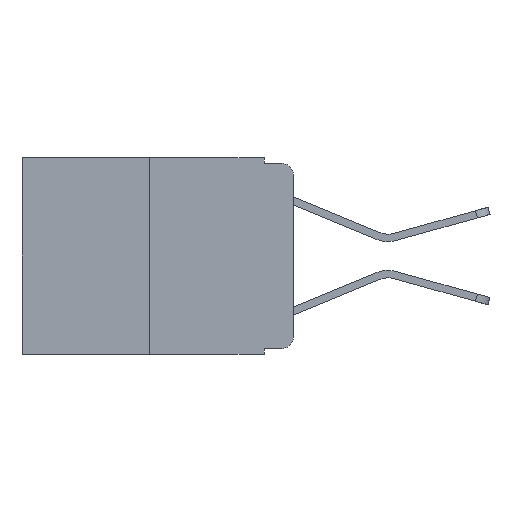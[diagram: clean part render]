
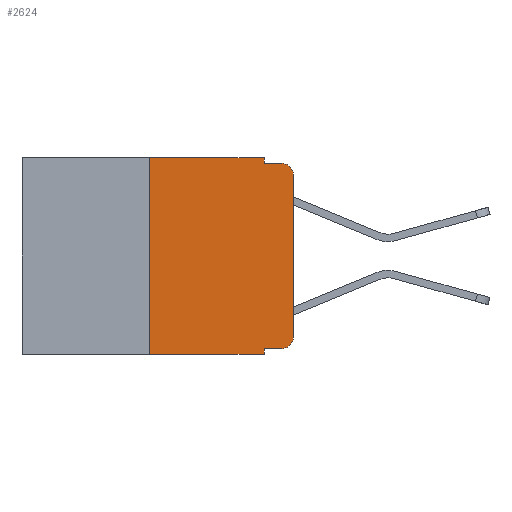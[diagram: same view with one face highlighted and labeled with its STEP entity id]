
A CAD part, left-side view. The second image highlights one B-rep face of the part: STEP entity #2624.
In plain terms, the highlighted planar face has unit normal (-1, 0, 0).
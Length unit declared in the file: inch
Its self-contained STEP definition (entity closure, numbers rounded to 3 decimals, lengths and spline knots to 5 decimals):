
#19 = ORIENTED_EDGE ( 'NONE', *, *, #8241, .F. ) ;
#22 = VECTOR ( 'NONE', #1344, 39.37008 ) ;
#104 = DIRECTION ( 'NONE',  ( 0., 0., -1. ) ) ;
#191 = ORIENTED_EDGE ( 'NONE', *, *, #8265, .F. ) ;
#260 = VERTEX_POINT ( 'NONE', #2706 ) ;
#266 = AXIS2_PLACEMENT_3D ( 'NONE', #10772, #7890, #8023 ) ;
#267 = VERTEX_POINT ( 'NONE', #2724 ) ;
#391 = LINE ( 'NONE', #6161, #5892 ) ;
#557 = ORIENTED_EDGE ( 'NONE', *, *, #8299, .T. ) ;
#726 = LINE ( 'NONE', #6759, #3659 ) ;
#813 = VERTEX_POINT ( 'NONE', #11244 ) ;
#1041 = FACE_OUTER_BOUND ( 'NONE', #6164, .T. ) ;
#1208 = CARTESIAN_POINT ( 'NONE',  ( 0., 0.25, 0. ) ) ;
#1344 = DIRECTION ( 'NONE',  ( 0., 0., 1. ) ) ;
#1414 = VECTOR ( 'NONE', #2322, 39.37008 ) ;
#1485 = EDGE_CURVE ( 'NONE', #267, #6537, #5308, .T. ) ;
#2110 = LINE ( 'NONE', #6670, #7257 ) ;
#2287 = VECTOR ( 'NONE', #10143, 39.37008 ) ;
#2322 = DIRECTION ( 'NONE',  ( 0., 0., 1. ) ) ;
#2362 = CARTESIAN_POINT ( 'NONE',  ( 0., 0.02, -0.313 ) ) ;
#2624 = ADVANCED_FACE ( 'NONE', ( #1041 ), #6940, .F. ) ;
#2632 = LINE ( 'NONE', #9280, #2287 ) ;
#2706 = CARTESIAN_POINT ( 'NONE',  ( 0., 0.02, -0.333 ) ) ;
#2724 = CARTESIAN_POINT ( 'NONE',  ( 0., 0., -0.03 ) ) ;
#3321 = LINE ( 'NONE', #7862, #22 ) ;
#3484 = DIRECTION ( 'NONE',  ( 0., 0., -1. ) ) ;
#3659 = VECTOR ( 'NONE', #9724, 39.37008 ) ;
#4106 = CARTESIAN_POINT ( 'NONE',  ( 0., 0.051, -0.01 ) ) ;
#4339 = CIRCLE ( 'NONE', #9671, 0.02 ) ;
#4487 = DIRECTION ( 'NONE',  ( 1., 0., 0. ) ) ;
#4524 = CARTESIAN_POINT ( 'NONE',  ( 0., 0.051, -0.01 ) ) ;
#4735 = VERTEX_POINT ( 'NONE', #4106 ) ;
#4807 = ORIENTED_EDGE ( 'NONE', *, *, #8283, .T. ) ;
#4826 = VERTEX_POINT ( 'NONE', #10610 ) ;
#5308 = CIRCLE ( 'NONE', #266, 0.02 ) ;
#5641 = DIRECTION ( 'NONE',  ( 0., 0., -1. ) ) ;
#5876 = ORIENTED_EDGE ( 'NONE', *, *, #8017, .F. ) ;
#5892 = VECTOR ( 'NONE', #7277, 39.37008 ) ;
#6161 = CARTESIAN_POINT ( 'NONE',  ( 0., 0.473, 0. ) ) ;
#6164 = EDGE_LOOP ( 'NONE', ( #557, #8243, #6881, #6557, #5876, #19, #9090, #191, #4807, #10189 ) ) ;
#6255 = CARTESIAN_POINT ( 'NONE',  ( 0., 0.02, -0.01 ) ) ;
#6537 = VERTEX_POINT ( 'NONE', #6255 ) ;
#6557 = ORIENTED_EDGE ( 'NONE', *, *, #8238, .F. ) ;
#6670 = CARTESIAN_POINT ( 'NONE',  ( 0., 0.051, 0. ) ) ;
#6759 = CARTESIAN_POINT ( 'NONE',  ( 0., 0.051, -0.333 ) ) ;
#6881 = ORIENTED_EDGE ( 'NONE', *, *, #8260, .F. ) ;
#6885 = LINE ( 'NONE', #4524, #9540 ) ;
#6940 = PLANE ( 'NONE',  #10767 ) ;
#7257 = VECTOR ( 'NONE', #104, 39.37008 ) ;
#7277 = DIRECTION ( 'NONE',  ( 0., -1., 0. ) ) ;
#7862 = CARTESIAN_POINT ( 'NONE',  ( 0., 0., 0. ) ) ;
#7890 = DIRECTION ( 'NONE',  ( -1., 0., 0. ) ) ;
#7990 = DIRECTION ( 'NONE',  ( 0., 0., -1. ) ) ;
#8017 = EDGE_CURVE ( 'NONE', #4826, #12088, #391, .T. ) ;
#8023 = DIRECTION ( 'NONE',  ( 0., 0., -1. ) ) ;
#8238 = EDGE_CURVE ( 'NONE', #12088, #4735, #2110, .T. ) ;
#8241 = EDGE_CURVE ( 'NONE', #9831, #4826, #12064, .T. ) ;
#8243 = ORIENTED_EDGE ( 'NONE', *, *, #1485, .T. ) ;
#8260 = EDGE_CURVE ( 'NONE', #4735, #6537, #6885, .T. ) ;
#8261 = EDGE_CURVE ( 'NONE', #260, #813, #4339, .T. ) ;
#8265 = EDGE_CURVE ( 'NONE', #9015, #10348, #9795, .T. ) ;
#8283 = EDGE_CURVE ( 'NONE', #9015, #260, #726, .T. ) ;
#8294 = CARTESIAN_POINT ( 'NONE',  ( 0., 0.051, -0.343 ) ) ;
#8299 = EDGE_CURVE ( 'NONE', #813, #267, #3321, .T. ) ;
#8480 = EDGE_CURVE ( 'NONE', #9831, #10348, #2632, .T. ) ;
#8798 = CARTESIAN_POINT ( 'NONE',  ( 0., 0.051, 0. ) ) ;
#9015 = VERTEX_POINT ( 'NONE', #12220 ) ;
#9090 = ORIENTED_EDGE ( 'NONE', *, *, #8480, .T. ) ;
#9258 = VECTOR ( 'NONE', #5641, 39.37008 ) ;
#9280 = CARTESIAN_POINT ( 'NONE',  ( 0., 0.473, -0.343 ) ) ;
#9540 = VECTOR ( 'NONE', #9664, 39.37008 ) ;
#9664 = DIRECTION ( 'NONE',  ( 0., -1., 0. ) ) ;
#9671 = AXIS2_PLACEMENT_3D ( 'NONE', #2362, #9694, #3484 ) ;
#9694 = DIRECTION ( 'NONE',  ( -1., 0., 0. ) ) ;
#9724 = DIRECTION ( 'NONE',  ( 0., -1., 0. ) ) ;
#9795 = LINE ( 'NONE', #8798, #9258 ) ;
#9831 = VERTEX_POINT ( 'NONE', #12698 ) ;
#10143 = DIRECTION ( 'NONE',  ( 0., -1., 0. ) ) ;
#10189 = ORIENTED_EDGE ( 'NONE', *, *, #8261, .T. ) ;
#10348 = VERTEX_POINT ( 'NONE', #8294 ) ;
#10610 = CARTESIAN_POINT ( 'NONE',  ( 0., 0.25, 0. ) ) ;
#10767 = AXIS2_PLACEMENT_3D ( 'NONE', #11044, #4487, #7990 ) ;
#10772 = CARTESIAN_POINT ( 'NONE',  ( 0., 0.02, -0.03 ) ) ;
#11044 = CARTESIAN_POINT ( 'NONE',  ( 0., 0.473, 0. ) ) ;
#11127 = CARTESIAN_POINT ( 'NONE',  ( 0., 0.051, 0. ) ) ;
#11244 = CARTESIAN_POINT ( 'NONE',  ( 0., 0., -0.313 ) ) ;
#12064 = LINE ( 'NONE', #1208, #1414 ) ;
#12088 = VERTEX_POINT ( 'NONE', #11127 ) ;
#12220 = CARTESIAN_POINT ( 'NONE',  ( 0., 0.051, -0.333 ) ) ;
#12698 = CARTESIAN_POINT ( 'NONE',  ( 0., 0.25, -0.343 ) ) ;
